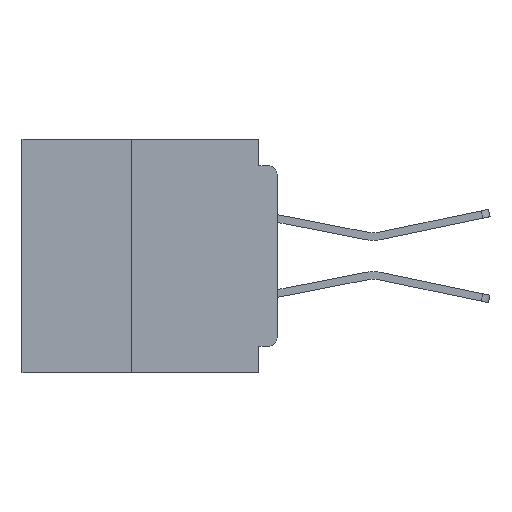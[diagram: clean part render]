
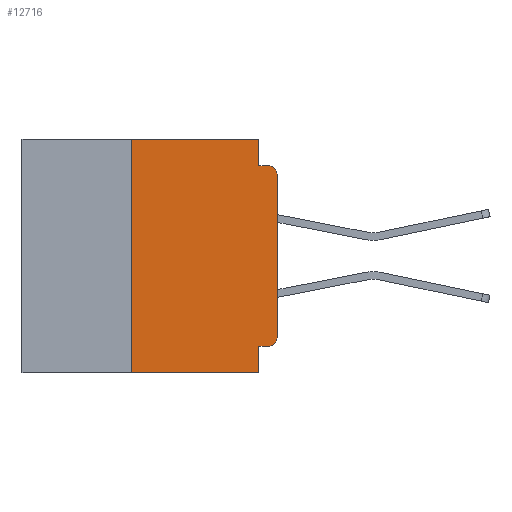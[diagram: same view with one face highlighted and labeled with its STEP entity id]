
A CAD part, left-side view. The second image highlights one B-rep face of the part: STEP entity #12716.
In plain terms, the highlighted planar face has unit normal (-1, 0, 0).
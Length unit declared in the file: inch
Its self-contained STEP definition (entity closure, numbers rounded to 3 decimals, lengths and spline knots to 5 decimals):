
#41 = CARTESIAN_POINT ( 'NONE',  ( 0., 0., -0.06 ) ) ;
#174 = PLANE ( 'NONE',  #24936 ) ;
#192 = VECTOR ( 'NONE', #21968, 39.37008 ) ;
#1281 = VERTEX_POINT ( 'NONE', #33828 ) ;
#1804 = DIRECTION ( 'NONE',  ( 0., 0., -1. ) ) ;
#1872 = VECTOR ( 'NONE', #23750, 39.37008 ) ;
#2038 = DIRECTION ( 'NONE',  ( -1., 0., 0. ) ) ;
#2129 = ORIENTED_EDGE ( 'NONE', *, *, #22934, .T. ) ;
#3612 = VERTEX_POINT ( 'NONE', #6356 ) ;
#4221 = VECTOR ( 'NONE', #28545, 39.37008 ) ;
#4966 = DIRECTION ( 'NONE',  ( 0., -1., 0. ) ) ;
#5969 = CARTESIAN_POINT ( 'NONE',  ( 0., 0.25, -0.4 ) ) ;
#6160 = ORIENTED_EDGE ( 'NONE', *, *, #12242, .F. ) ;
#6356 = CARTESIAN_POINT ( 'NONE',  ( 0., 0.031, -0.4 ) ) ;
#8178 = VECTOR ( 'NONE', #4966, 39.37008 ) ;
#9132 = DIRECTION ( 'NONE',  ( 1., 0., 0. ) ) ;
#9195 = LINE ( 'NONE', #15593, #24069 ) ;
#10141 = CARTESIAN_POINT ( 'NONE',  ( 0., 0., -0.355 ) ) ;
#10183 = VERTEX_POINT ( 'NONE', #14559 ) ;
#10226 = VECTOR ( 'NONE', #18253, 39.37008 ) ;
#11329 = ORIENTED_EDGE ( 'NONE', *, *, #16612, .F. ) ;
#11902 = ORIENTED_EDGE ( 'NONE', *, *, #15214, .F. ) ;
#12242 = EDGE_CURVE ( 'NONE', #30511, #1281, #15958, .T. ) ;
#12716 = ADVANCED_FACE ( 'NONE', ( #14993 ), #174, .F. ) ;
#13024 = LINE ( 'NONE', #24279, #10226 ) ;
#13537 = CARTESIAN_POINT ( 'NONE',  ( 0., 0.25, -0.4 ) ) ;
#13869 = VERTEX_POINT ( 'NONE', #35592 ) ;
#14559 = CARTESIAN_POINT ( 'NONE',  ( 0., 0.031, 0. ) ) ;
#14993 = FACE_OUTER_BOUND ( 'NONE', #34950, .T. ) ;
#15214 = EDGE_CURVE ( 'NONE', #10183, #22656, #13024, .T. ) ;
#15593 = CARTESIAN_POINT ( 'NONE',  ( 0., 0.437, 0. ) ) ;
#15958 = LINE ( 'NONE', #10141, #192 ) ;
#16164 = CIRCLE ( 'NONE', #38168, 0.015 ) ;
#16181 = EDGE_CURVE ( 'NONE', #35332, #17410, #16164, .T. ) ;
#16612 = EDGE_CURVE ( 'NONE', #13869, #10183, #9195, .T. ) ;
#17281 = ORIENTED_EDGE ( 'NONE', *, *, #29152, .F. ) ;
#17410 = VERTEX_POINT ( 'NONE', #31201 ) ;
#17599 = LINE ( 'NONE', #5969, #1872 ) ;
#17925 = CARTESIAN_POINT ( 'NONE',  ( 0., 0.437, 0. ) ) ;
#18253 = DIRECTION ( 'NONE',  ( 0., 0., -1. ) ) ;
#18825 = VECTOR ( 'NONE', #35329, 39.37008 ) ;
#19528 = DIRECTION ( 'NONE',  ( -1., 0., 0. ) ) ;
#19761 = CARTESIAN_POINT ( 'NONE',  ( 0., 0.015, -0.34 ) ) ;
#20234 = VERTEX_POINT ( 'NONE', #13537 ) ;
#20365 = AXIS2_PLACEMENT_3D ( 'NONE', #19761, #2038, #22782 ) ;
#21290 = CARTESIAN_POINT ( 'NONE',  ( 0., 0.031, -0.4 ) ) ;
#21592 = DIRECTION ( 'NONE',  ( 0., -1., 0. ) ) ;
#21968 = DIRECTION ( 'NONE',  ( 0., 1., 0. ) ) ;
#22173 = VERTEX_POINT ( 'NONE', #24716 ) ;
#22656 = VERTEX_POINT ( 'NONE', #32880 ) ;
#22782 = DIRECTION ( 'NONE',  ( 0., 0., -1. ) ) ;
#22934 = EDGE_CURVE ( 'NONE', #22173, #35332, #34670, .T. ) ;
#23214 = EDGE_CURVE ( 'NONE', #20234, #13869, #17599, .T. ) ;
#23724 = CARTESIAN_POINT ( 'NONE',  ( 0., 0., -0.045 ) ) ;
#23750 = DIRECTION ( 'NONE',  ( 0., 0., 1. ) ) ;
#24069 = VECTOR ( 'NONE', #21592, 39.37008 ) ;
#24184 = EDGE_CURVE ( 'NONE', #30511, #22173, #36349, .T. ) ;
#24279 = CARTESIAN_POINT ( 'NONE',  ( 0., 0.031, 0. ) ) ;
#24716 = CARTESIAN_POINT ( 'NONE',  ( 0., 0., -0.34 ) ) ;
#24838 = ORIENTED_EDGE ( 'NONE', *, *, #23214, .F. ) ;
#24936 = AXIS2_PLACEMENT_3D ( 'NONE', #17925, #9132, #29867 ) ;
#25187 = EDGE_CURVE ( 'NONE', #20234, #3612, #25828, .T. ) ;
#25580 = CARTESIAN_POINT ( 'NONE',  ( 0., 0., 0. ) ) ;
#25705 = CARTESIAN_POINT ( 'NONE',  ( 0., 0.437, -0.4 ) ) ;
#25828 = LINE ( 'NONE', #25705, #8178 ) ;
#25887 = LINE ( 'NONE', #21290, #30926 ) ;
#27194 = CARTESIAN_POINT ( 'NONE',  ( 0., 0.015, -0.355 ) ) ;
#28545 = DIRECTION ( 'NONE',  ( 0., 0., 1. ) ) ;
#29152 = EDGE_CURVE ( 'NONE', #1281, #3612, #25887, .T. ) ;
#29702 = ORIENTED_EDGE ( 'NONE', *, *, #24184, .T. ) ;
#29867 = DIRECTION ( 'NONE',  ( 0., 0., -1. ) ) ;
#30223 = DIRECTION ( 'NONE',  ( 0., 0., -1. ) ) ;
#30511 = VERTEX_POINT ( 'NONE', #27194 ) ;
#30926 = VECTOR ( 'NONE', #30223, 39.37008 ) ;
#31201 = CARTESIAN_POINT ( 'NONE',  ( 0., 0.015, -0.045 ) ) ;
#32880 = CARTESIAN_POINT ( 'NONE',  ( 0., 0.031, -0.045 ) ) ;
#33828 = CARTESIAN_POINT ( 'NONE',  ( 0., 0.031, -0.355 ) ) ;
#33916 = ORIENTED_EDGE ( 'NONE', *, *, #16181, .T. ) ;
#34492 = LINE ( 'NONE', #23724, #18825 ) ;
#34670 = LINE ( 'NONE', #25580, #4221 ) ;
#34682 = EDGE_CURVE ( 'NONE', #22656, #17410, #34492, .T. ) ;
#34831 = ORIENTED_EDGE ( 'NONE', *, *, #25187, .T. ) ;
#34950 = EDGE_LOOP ( 'NONE', ( #2129, #33916, #36535, #11902, #11329, #24838, #34831, #17281, #6160, #29702 ) ) ;
#35329 = DIRECTION ( 'NONE',  ( 0., -1., 0. ) ) ;
#35332 = VERTEX_POINT ( 'NONE', #41 ) ;
#35592 = CARTESIAN_POINT ( 'NONE',  ( 0., 0.25, 0. ) ) ;
#36349 = CIRCLE ( 'NONE', #20365, 0.015 ) ;
#36535 = ORIENTED_EDGE ( 'NONE', *, *, #34682, .F. ) ;
#37060 = CARTESIAN_POINT ( 'NONE',  ( 0., 0.015, -0.06 ) ) ;
#38168 = AXIS2_PLACEMENT_3D ( 'NONE', #37060, #19528, #1804 ) ;
